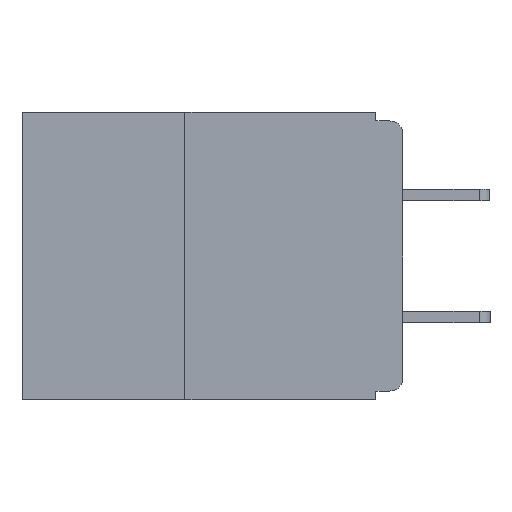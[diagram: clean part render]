
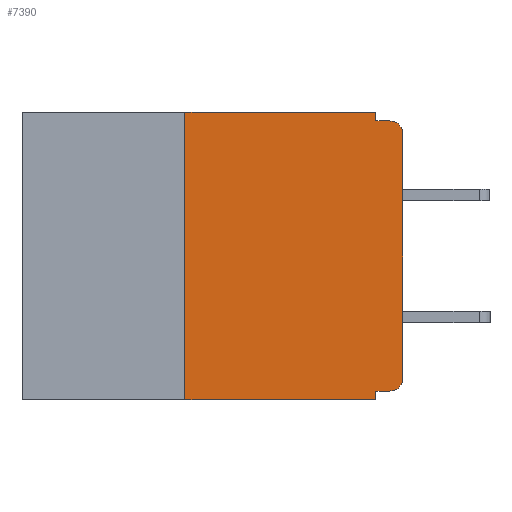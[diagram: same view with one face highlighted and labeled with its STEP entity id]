
A CAD part, left-side view. The second image highlights one B-rep face of the part: STEP entity #7390.
In plain terms, the highlighted planar face has unit normal (-1, 0, 0).
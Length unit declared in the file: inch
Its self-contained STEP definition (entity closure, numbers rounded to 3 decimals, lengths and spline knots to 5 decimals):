
#243 = VECTOR ( 'NONE', #5052, 39.37008 ) ;
#309 = DIRECTION ( 'NONE',  ( 0., 0., -1. ) ) ;
#385 = LINE ( 'NONE', #7904, #15854 ) ;
#676 = DIRECTION ( 'NONE',  ( 0., 0., -1. ) ) ;
#694 = DIRECTION ( 'NONE',  ( -1., 0., 0. ) ) ;
#696 = CARTESIAN_POINT ( 'NONE',  ( 0., 0.015, -0.025 ) ) ;
#830 = CIRCLE ( 'NONE', #17930, 0.015 ) ;
#1274 = FACE_OUTER_BOUND ( 'NONE', #14123, .T. ) ;
#1441 = VECTOR ( 'NONE', #7396, 39.37008 ) ;
#1473 = VECTOR ( 'NONE', #10603, 39.37008 ) ;
#1731 = ORIENTED_EDGE ( 'NONE', *, *, #11756, .T. ) ;
#2199 = VECTOR ( 'NONE', #15090, 39.37008 ) ;
#2210 = ORIENTED_EDGE ( 'NONE', *, *, #8983, .F. ) ;
#2348 = CARTESIAN_POINT ( 'NONE',  ( 0., 0.031, 0. ) ) ;
#2501 = CIRCLE ( 'NONE', #13933, 0.015 ) ;
#2647 = CARTESIAN_POINT ( 'NONE',  ( 0., 0.015, -0.32 ) ) ;
#3364 = ORIENTED_EDGE ( 'NONE', *, *, #10891, .T. ) ;
#3453 = VECTOR ( 'NONE', #6271, 39.37008 ) ;
#3612 = VERTEX_POINT ( 'NONE', #2647 ) ;
#3759 = EDGE_CURVE ( 'NONE', #16727, #7637, #830, .T. ) ;
#3930 = LINE ( 'NONE', #13385, #3453 ) ;
#4101 = EDGE_CURVE ( 'NONE', #4294, #10790, #6174, .T. ) ;
#4294 = VERTEX_POINT ( 'NONE', #12865 ) ;
#4720 = CARTESIAN_POINT ( 'NONE',  ( 0., 0.031, -0.33 ) ) ;
#4793 = VERTEX_POINT ( 'NONE', #6441 ) ;
#5052 = DIRECTION ( 'NONE',  ( 0., -1., 0. ) ) ;
#5282 = ORIENTED_EDGE ( 'NONE', *, *, #9254, .F. ) ;
#5287 = CARTESIAN_POINT ( 'NONE',  ( 0., 0.031, -0.01 ) ) ;
#6089 = EDGE_CURVE ( 'NONE', #4294, #7033, #9137, .T. ) ;
#6174 = LINE ( 'NONE', #15180, #2199 ) ;
#6271 = DIRECTION ( 'NONE',  ( 0., 1., 0. ) ) ;
#6441 = CARTESIAN_POINT ( 'NONE',  ( 0., 0., -0.305 ) ) ;
#6729 = DIRECTION ( 'NONE',  ( 0., 0., 1. ) ) ;
#6836 = ORIENTED_EDGE ( 'NONE', *, *, #6089, .F. ) ;
#7033 = VERTEX_POINT ( 'NONE', #8044 ) ;
#7390 = ADVANCED_FACE ( 'NONE', ( #1274 ), #17449, .F. ) ;
#7396 = DIRECTION ( 'NONE',  ( 0., 0., -1. ) ) ;
#7637 = VERTEX_POINT ( 'NONE', #14892 ) ;
#7683 = DIRECTION ( 'NONE',  ( 0., 0., 1. ) ) ;
#7874 = CARTESIAN_POINT ( 'NONE',  ( 0., 0.25, -0.33 ) ) ;
#7904 = CARTESIAN_POINT ( 'NONE',  ( 0., 0.031, -0.33 ) ) ;
#8044 = CARTESIAN_POINT ( 'NONE',  ( 0., 0.25, 0. ) ) ;
#8061 = EDGE_CURVE ( 'NONE', #7033, #16136, #9297, .T. ) ;
#8080 = VECTOR ( 'NONE', #6729, 39.37008 ) ;
#8983 = EDGE_CURVE ( 'NONE', #16136, #10504, #15959, .T. ) ;
#9110 = ORIENTED_EDGE ( 'NONE', *, *, #3759, .T. ) ;
#9137 = LINE ( 'NONE', #7874, #18575 ) ;
#9161 = DIRECTION ( 'NONE',  ( -1., 0., 0. ) ) ;
#9254 = EDGE_CURVE ( 'NONE', #10504, #7637, #14819, .T. ) ;
#9297 = LINE ( 'NONE', #10640, #1473 ) ;
#10504 = VERTEX_POINT ( 'NONE', #5287 ) ;
#10603 = DIRECTION ( 'NONE',  ( 0., -1., 0. ) ) ;
#10640 = CARTESIAN_POINT ( 'NONE',  ( 0., 0.437, 0. ) ) ;
#10790 = VERTEX_POINT ( 'NONE', #4720 ) ;
#10891 = EDGE_CURVE ( 'NONE', #3612, #4793, #2501, .T. ) ;
#11561 = ORIENTED_EDGE ( 'NONE', *, *, #8061, .F. ) ;
#11756 = EDGE_CURVE ( 'NONE', #4793, #16727, #15654, .T. ) ;
#12478 = EDGE_CURVE ( 'NONE', #3612, #15117, #3930, .T. ) ;
#12494 = CARTESIAN_POINT ( 'NONE',  ( 0., 0., 0. ) ) ;
#12865 = CARTESIAN_POINT ( 'NONE',  ( 0., 0.25, -0.33 ) ) ;
#13385 = CARTESIAN_POINT ( 'NONE',  ( 0., 0., -0.32 ) ) ;
#13891 = CARTESIAN_POINT ( 'NONE',  ( 0., 0., -0.025 ) ) ;
#13933 = AXIS2_PLACEMENT_3D ( 'NONE', #17613, #9161, #309 ) ;
#14123 = EDGE_LOOP ( 'NONE', ( #1731, #9110, #5282, #2210, #11561, #6836, #14896, #18272, #18372, #3364 ) ) ;
#14364 = AXIS2_PLACEMENT_3D ( 'NONE', #17819, #17359, #17340 ) ;
#14510 = CARTESIAN_POINT ( 'NONE',  ( 0., 0.031, 0. ) ) ;
#14819 = LINE ( 'NONE', #16492, #243 ) ;
#14892 = CARTESIAN_POINT ( 'NONE',  ( 0., 0.015, -0.01 ) ) ;
#14896 = ORIENTED_EDGE ( 'NONE', *, *, #4101, .T. ) ;
#15090 = DIRECTION ( 'NONE',  ( 0., -1., 0. ) ) ;
#15117 = VERTEX_POINT ( 'NONE', #16009 ) ;
#15180 = CARTESIAN_POINT ( 'NONE',  ( 0., 0.437, -0.33 ) ) ;
#15654 = LINE ( 'NONE', #12494, #8080 ) ;
#15854 = VECTOR ( 'NONE', #17791, 39.37008 ) ;
#15959 = LINE ( 'NONE', #14510, #1441 ) ;
#16009 = CARTESIAN_POINT ( 'NONE',  ( 0., 0.031, -0.32 ) ) ;
#16136 = VERTEX_POINT ( 'NONE', #2348 ) ;
#16492 = CARTESIAN_POINT ( 'NONE',  ( 0., 0., -0.01 ) ) ;
#16727 = VERTEX_POINT ( 'NONE', #13891 ) ;
#17340 = DIRECTION ( 'NONE',  ( 0., 0., -1. ) ) ;
#17359 = DIRECTION ( 'NONE',  ( 1., 0., 0. ) ) ;
#17449 = PLANE ( 'NONE',  #14364 ) ;
#17613 = CARTESIAN_POINT ( 'NONE',  ( 0., 0.015, -0.305 ) ) ;
#17791 = DIRECTION ( 'NONE',  ( 0., 0., -1. ) ) ;
#17819 = CARTESIAN_POINT ( 'NONE',  ( 0., 0.437, 0. ) ) ;
#17851 = EDGE_CURVE ( 'NONE', #15117, #10790, #385, .T. ) ;
#17930 = AXIS2_PLACEMENT_3D ( 'NONE', #696, #694, #676 ) ;
#18272 = ORIENTED_EDGE ( 'NONE', *, *, #17851, .F. ) ;
#18372 = ORIENTED_EDGE ( 'NONE', *, *, #12478, .F. ) ;
#18575 = VECTOR ( 'NONE', #7683, 39.37008 ) ;
